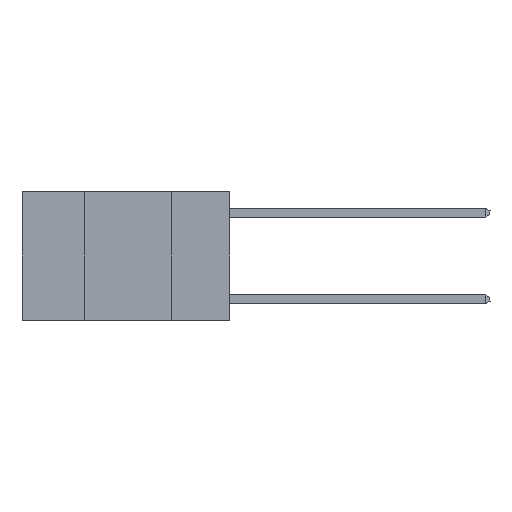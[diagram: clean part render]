
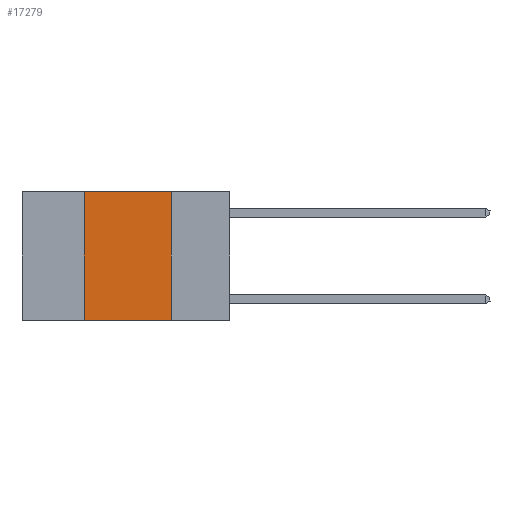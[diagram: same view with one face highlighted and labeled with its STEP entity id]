
A CAD part, left-side view. The second image highlights one B-rep face of the part: STEP entity #17279.
In plain terms, the highlighted planar face has unit normal (-1, 0, 0).
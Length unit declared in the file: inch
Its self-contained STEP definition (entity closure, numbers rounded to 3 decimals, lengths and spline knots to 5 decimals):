
#1061 = VERTEX_POINT ( 'NONE', #19529 ) ;
#1304 = EDGE_CURVE ( 'NONE', #16498, #12976, #12968, .T. ) ;
#1359 = CARTESIAN_POINT ( 'NONE',  ( 0., 0.42, 0. ) ) ;
#2447 = AXIS2_PLACEMENT_3D ( 'NONE', #6784, #12805, #4414 ) ;
#3724 = CARTESIAN_POINT ( 'NONE',  ( 0., 0.17, 0. ) ) ;
#4414 = DIRECTION ( 'NONE',  ( 0., 0., -1. ) ) ;
#5269 = DIRECTION ( 'NONE',  ( 0., 0., 1. ) ) ;
#5779 = CARTESIAN_POINT ( 'NONE',  ( 0., 0.6, -0.37 ) ) ;
#6784 = CARTESIAN_POINT ( 'NONE',  ( 0., 0.6, 0. ) ) ;
#8157 = LINE ( 'NONE', #5779, #16766 ) ;
#8208 = CARTESIAN_POINT ( 'NONE',  ( 0., 0.6, 0. ) ) ;
#8376 = ORIENTED_EDGE ( 'NONE', *, *, #20720, .F. ) ;
#8507 = VERTEX_POINT ( 'NONE', #22327 ) ;
#9700 = VECTOR ( 'NONE', #12248, 39.37008 ) ;
#12063 = EDGE_CURVE ( 'NONE', #8507, #16498, #24412, .T. ) ;
#12248 = DIRECTION ( 'NONE',  ( 0., 0., -1. ) ) ;
#12805 = DIRECTION ( 'NONE',  ( 1., 0., 0. ) ) ;
#12968 = LINE ( 'NONE', #8208, #24330 ) ;
#12976 = VERTEX_POINT ( 'NONE', #15676 ) ;
#15676 = CARTESIAN_POINT ( 'NONE',  ( 0., 0.17, 0. ) ) ;
#16498 = VERTEX_POINT ( 'NONE', #18398 ) ;
#16766 = VECTOR ( 'NONE', #18614, 39.37008 ) ;
#16983 = FACE_OUTER_BOUND ( 'NONE', #17499, .T. ) ;
#17279 = ADVANCED_FACE ( 'NONE', ( #16983 ), #17515, .F. ) ;
#17499 = EDGE_LOOP ( 'NONE', ( #8376, #18312, #22571, #19183 ) ) ;
#17515 = PLANE ( 'NONE',  #2447 ) ;
#18312 = ORIENTED_EDGE ( 'NONE', *, *, #1304, .F. ) ;
#18398 = CARTESIAN_POINT ( 'NONE',  ( 0., 0.42, 0. ) ) ;
#18614 = DIRECTION ( 'NONE',  ( 0., -1., 0. ) ) ;
#18844 = EDGE_CURVE ( 'NONE', #8507, #1061, #8157, .T. ) ;
#19083 = DIRECTION ( 'NONE',  ( 0., -1., 0. ) ) ;
#19183 = ORIENTED_EDGE ( 'NONE', *, *, #18844, .T. ) ;
#19529 = CARTESIAN_POINT ( 'NONE',  ( 0., 0.17, -0.37 ) ) ;
#19671 = VECTOR ( 'NONE', #5269, 39.37008 ) ;
#20720 = EDGE_CURVE ( 'NONE', #12976, #1061, #20722, .T. ) ;
#20722 = LINE ( 'NONE', #3724, #9700 ) ;
#22327 = CARTESIAN_POINT ( 'NONE',  ( 0., 0.42, -0.37 ) ) ;
#22571 = ORIENTED_EDGE ( 'NONE', *, *, #12063, .F. ) ;
#24330 = VECTOR ( 'NONE', #19083, 39.37008 ) ;
#24412 = LINE ( 'NONE', #1359, #19671 ) ;
